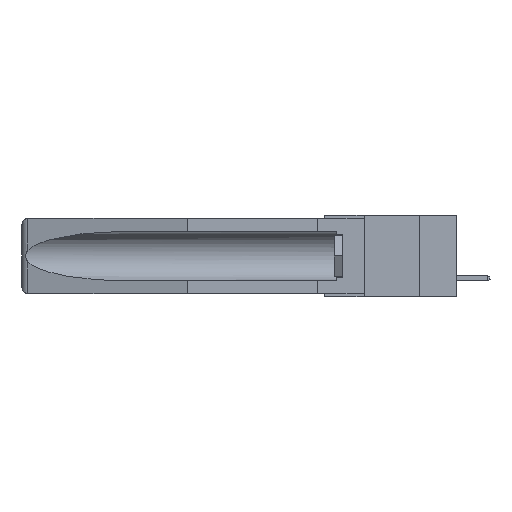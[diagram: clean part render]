
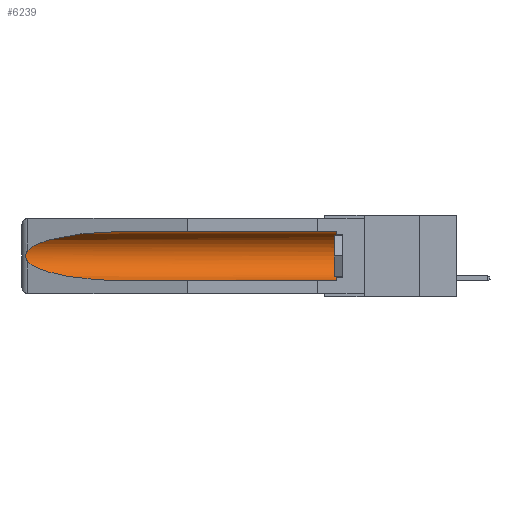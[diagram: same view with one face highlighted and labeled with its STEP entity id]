
A CAD part, left-side view. The second image highlights one B-rep face of the part: STEP entity #6239.
In plain terms, the highlighted cylindrical face has radius 2.857 mm (diameter 5.715 mm), a partial arc.
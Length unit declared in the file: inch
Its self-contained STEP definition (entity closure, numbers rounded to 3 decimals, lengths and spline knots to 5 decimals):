
#55 =( BOUNDED_CURVE ( )  B_SPLINE_CURVE ( 3, ( #1761, #7132, #8528, #4492 ),
 .UNSPECIFIED., .F., .T. ) 
 B_SPLINE_CURVE_WITH_KNOTS ( ( 4, 4 ),
 ( 0.1948, 1.5708 ),
 .UNSPECIFIED. ) 
 CURVE ( )  GEOMETRIC_REPRESENTATION_ITEM ( )  RATIONAL_B_SPLINE_CURVE ( ( 1., 0.848, 0.848, 1. ) ) 
 REPRESENTATION_ITEM ( '' )  );
#73 = LINE ( 'NONE', #8739, #12596 ) ;
#144 = DIRECTION ( 'NONE',  ( 0., 1., 0. ) ) ;
#305 = FACE_OUTER_BOUND ( 'NONE', #13586, .T. ) ;
#327 = CARTESIAN_POINT ( 'NONE',  ( 0.155, 0.126, -0.284 ) ) ;
#525 = DIRECTION ( 'NONE',  ( 0., -1., 0. ) ) ;
#797 = DIRECTION ( 'NONE',  ( 0., 1., 0. ) ) ;
#974 = VERTEX_POINT ( 'NONE', #327 ) ;
#998 = VERTEX_POINT ( 'NONE', #5572 ) ;
#1290 = B_SPLINE_CURVE_WITH_KNOTS ( 'NONE', 3,
 ( #2435, #10303, #11760, #15755, #13166, #5142, #11998, #6740, #14493, #6502 ),
 .UNSPECIFIED., .F., .F.,
 ( 4, 2, 2, 2, 4 ),
 ( 0., 0.00029, 0.00058, 0.00087, 0.00117 ),
 .UNSPECIFIED. ) ;
#1761 = CARTESIAN_POINT ( 'NONE',  ( 0.26537, 1.52718, -0.19328 ) ) ;
#2435 = CARTESIAN_POINT ( 'NONE',  ( 0.26537, 1.52718, -0.14972 ) ) ;
#2780 = CARTESIAN_POINT ( 'NONE',  ( 0.155, 1.07973, -0.284 ) ) ;
#3027 = CARTESIAN_POINT ( 'NONE',  ( 0.26537, 1.52718, -0.14972 ) ) ;
#4225 = ORIENTED_EDGE ( 'NONE', *, *, #14495, .T. ) ;
#4386 = CARTESIAN_POINT ( 'NONE',  ( 0.25451, 1.48313, -0.09465 ) ) ;
#4492 = CARTESIAN_POINT ( 'NONE',  ( 0.155, 1.07973, -0.284 ) ) ;
#4559 = CARTESIAN_POINT ( 'NONE',  ( 0.21114, 1.30732, -0.059 ) ) ;
#4762 = DIRECTION ( 'NONE',  ( 0., 0., 1. ) ) ;
#5142 = CARTESIAN_POINT ( 'NONE',  ( 0.2675, 1.53308, -0.17534 ) ) ;
#5292 = CYLINDRICAL_SURFACE ( 'NONE', #10021, 0.1125 ) ;
#5572 = CARTESIAN_POINT ( 'NONE',  ( 0.155, 1.07973, -0.059 ) ) ;
#5761 = EDGE_CURVE ( 'NONE', #12934, #16997, #55, .T. ) ;
#6183 = EDGE_CURVE ( 'NONE', #12953, #998, #6350, .T. ) ;
#6239 = ADVANCED_FACE ( 'NONE', ( #305 ), #5292, .F. ) ;
#6350 = LINE ( 'NONE', #11621, #8461 ) ;
#6395 = ORIENTED_EDGE ( 'NONE', *, *, #5761, .T. ) ;
#6502 = CARTESIAN_POINT ( 'NONE',  ( 0.26537, 1.52718, -0.19328 ) ) ;
#6740 = CARTESIAN_POINT ( 'NONE',  ( 0.26655, 1.53094, -0.18657 ) ) ;
#7132 = CARTESIAN_POINT ( 'NONE',  ( 0.25451, 1.48313, -0.24835 ) ) ;
#7266 = EDGE_CURVE ( 'NONE', #998, #15008, #10615, .T. ) ;
#7404 = CARTESIAN_POINT ( 'NONE',  ( 0.155, 0.126, -0.1715 ) ) ;
#7875 = CARTESIAN_POINT ( 'NONE',  ( 0.26537, 1.52718, -0.19328 ) ) ;
#8140 = CARTESIAN_POINT ( 'NONE',  ( 0.155, -0.30754, -0.1715 ) ) ;
#8280 = ORIENTED_EDGE ( 'NONE', *, *, #16727, .T. ) ;
#8461 = VECTOR ( 'NONE', #15625, 39.37008 ) ;
#8528 = CARTESIAN_POINT ( 'NONE',  ( 0.21114, 1.30732, -0.284 ) ) ;
#8739 = CARTESIAN_POINT ( 'NONE',  ( 0.155, -0.30754, -0.284 ) ) ;
#9147 = ORIENTED_EDGE ( 'NONE', *, *, #12171, .F. ) ;
#10021 = AXIS2_PLACEMENT_3D ( 'NONE', #8140, #144, #17246 ) ;
#10303 = CARTESIAN_POINT ( 'NONE',  ( 0.26597, 1.52961, -0.15275 ) ) ;
#10615 =( BOUNDED_CURVE ( )  B_SPLINE_CURVE ( 3, ( #16292, #4559, #4386, #11126 ),
 .UNSPECIFIED., .F., .F. ) 
 B_SPLINE_CURVE_WITH_KNOTS ( ( 4, 4 ),
 ( 4.71239, 6.08839 ),
 .UNSPECIFIED. ) 
 CURVE ( )  GEOMETRIC_REPRESENTATION_ITEM ( )  RATIONAL_B_SPLINE_CURVE ( ( 1., 0.848, 0.848, 1. ) ) 
 REPRESENTATION_ITEM ( '' )  );
#10633 = CIRCLE ( 'NONE', #14086, 0.1125 ) ;
#11126 = CARTESIAN_POINT ( 'NONE',  ( 0.26537, 1.52718, -0.14972 ) ) ;
#11621 = CARTESIAN_POINT ( 'NONE',  ( 0.155, -0.30754, -0.059 ) ) ;
#11760 = CARTESIAN_POINT ( 'NONE',  ( 0.26654, 1.53092, -0.15636 ) ) ;
#11998 = CARTESIAN_POINT ( 'NONE',  ( 0.2673, 1.53269, -0.17917 ) ) ;
#12171 = EDGE_CURVE ( 'NONE', #974, #16997, #73, .T. ) ;
#12596 = VECTOR ( 'NONE', #797, 39.37008 ) ;
#12934 = VERTEX_POINT ( 'NONE', #7875 ) ;
#12953 = VERTEX_POINT ( 'NONE', #14565 ) ;
#13166 = CARTESIAN_POINT ( 'NONE',  ( 0.2675, 1.53308, -0.16763 ) ) ;
#13512 = ORIENTED_EDGE ( 'NONE', *, *, #6183, .T. ) ;
#13586 = EDGE_LOOP ( 'NONE', ( #16064, #8280, #6395, #9147, #4225, #13512 ) ) ;
#14086 = AXIS2_PLACEMENT_3D ( 'NONE', #7404, #525, #4762 ) ;
#14493 = CARTESIAN_POINT ( 'NONE',  ( 0.26597, 1.5296, -0.19026 ) ) ;
#14495 = EDGE_CURVE ( 'NONE', #974, #12953, #10633, .T. ) ;
#14565 = CARTESIAN_POINT ( 'NONE',  ( 0.155, 0.126, -0.059 ) ) ;
#15008 = VERTEX_POINT ( 'NONE', #3027 ) ;
#15625 = DIRECTION ( 'NONE',  ( 0., 1., 0. ) ) ;
#15755 = CARTESIAN_POINT ( 'NONE',  ( 0.2673, 1.5327, -0.16383 ) ) ;
#16064 = ORIENTED_EDGE ( 'NONE', *, *, #7266, .T. ) ;
#16292 = CARTESIAN_POINT ( 'NONE',  ( 0.155, 1.07973, -0.059 ) ) ;
#16727 = EDGE_CURVE ( 'NONE', #15008, #12934, #1290, .T. ) ;
#16997 = VERTEX_POINT ( 'NONE', #2780 ) ;
#17246 = DIRECTION ( 'NONE',  ( 0., 0., 1. ) ) ;
